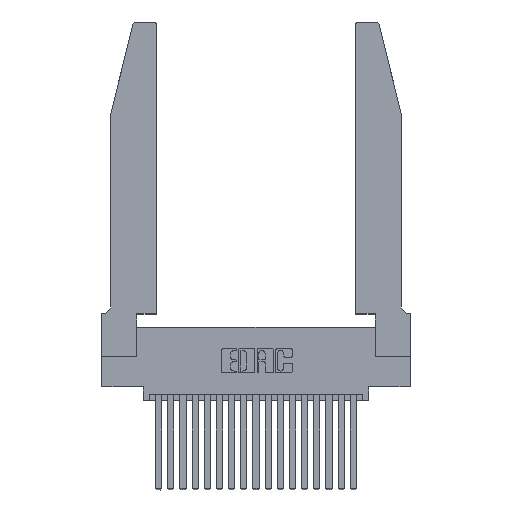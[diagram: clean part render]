
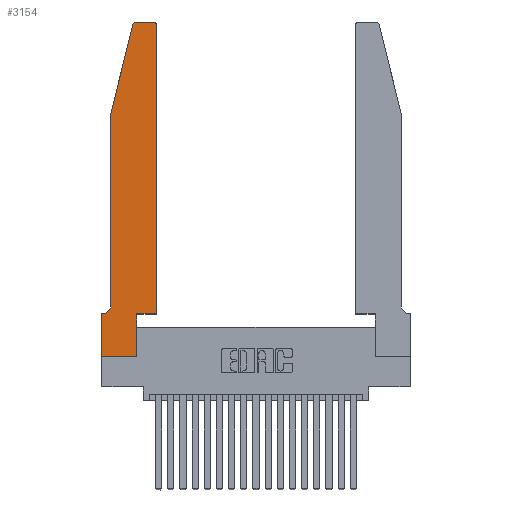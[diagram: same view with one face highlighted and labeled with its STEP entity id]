
A CAD part, top view. The second image highlights one B-rep face of the part: STEP entity #3154.
In plain terms, the highlighted planar face has unit normal (0, 0, 1).
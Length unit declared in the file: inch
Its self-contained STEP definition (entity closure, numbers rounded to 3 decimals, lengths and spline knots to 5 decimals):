
#36 = VECTOR ( 'NONE', #15393, 39.37008 ) ;
#44 = DIRECTION ( 'NONE',  ( 1., 0., 0. ) ) ;
#97 = CARTESIAN_POINT ( 'NONE',  ( 0.0055, 0.35, 0.37 ) ) ;
#299 = CIRCLE ( 'NONE', #5243, 0.07 ) ;
#672 = CARTESIAN_POINT ( 'NONE',  ( 0., 0., 0.37 ) ) ;
#752 = EDGE_CURVE ( 'NONE', #21136, #11259, #12921, .T. ) ;
#969 = CARTESIAN_POINT ( 'NONE',  ( 0.4505, 0.35, 0.37 ) ) ;
#1030 = VERTEX_POINT ( 'NONE', #6808 ) ;
#1181 = DIRECTION ( 'NONE',  ( 1., 0., 0. ) ) ;
#1696 = DIRECTION ( 'NONE',  ( 1., 0., 0. ) ) ;
#1903 = DIRECTION ( 'NONE',  ( -1., 0., 0. ) ) ;
#1952 = VECTOR ( 'NONE', #4539, 39.37008 ) ;
#2122 = VECTOR ( 'NONE', #17268, 39.37008 ) ;
#2132 = AXIS2_PLACEMENT_3D ( 'NONE', #18991, #7705, #6198 ) ;
#2528 = VECTOR ( 'NONE', #1696, 39.37008 ) ;
#2540 = CARTESIAN_POINT ( 'NONE',  ( 0.2865, 0., 0.37 ) ) ;
#2707 = LINE ( 'NONE', #16855, #19790 ) ;
#3154 = ADVANCED_FACE ( 'NONE', ( #4166 ), #10965, .T. ) ;
#3483 = DIRECTION ( 'NONE',  ( -1., 0., 0. ) ) ;
#3607 = VERTEX_POINT ( 'NONE', #16973 ) ;
#3768 = DIRECTION ( 'NONE',  ( 0., -1., 0. ) ) ;
#4088 = LINE ( 'NONE', #9942, #2528 ) ;
#4166 = FACE_OUTER_BOUND ( 'NONE', #20637, .T. ) ;
#4196 = VECTOR ( 'NONE', #15660, 39.37008 ) ;
#4365 = ORIENTED_EDGE ( 'NONE', *, *, #20532, .T. ) ;
#4539 = DIRECTION ( 'NONE',  ( -0.239, -0.971, 0. ) ) ;
#4566 = DIRECTION ( 'NONE',  ( 0., 0., 1. ) ) ;
#4737 = CARTESIAN_POINT ( 'NONE',  ( 0.4505, 0.35, 0.37 ) ) ;
#4977 = LINE ( 'NONE', #672, #4196 ) ;
#5243 = AXIS2_PLACEMENT_3D ( 'NONE', #11735, #13390, #3483 ) ;
#5324 = VECTOR ( 'NONE', #1903, 39.37008 ) ;
#5449 = ORIENTED_EDGE ( 'NONE', *, *, #10488, .T. ) ;
#5749 = VERTEX_POINT ( 'NONE', #17830 ) ;
#5934 = CARTESIAN_POINT ( 'NONE',  ( 0.25487, 2.72718, 0.37 ) ) ;
#6198 = DIRECTION ( 'NONE',  ( 1., 0., 0. ) ) ;
#6441 = ORIENTED_EDGE ( 'NONE', *, *, #20755, .T. ) ;
#6808 = CARTESIAN_POINT ( 'NONE',  ( 0.0755, 2., 0.37 ) ) ;
#7166 = CARTESIAN_POINT ( 'NONE',  ( 0.0755, 2., 0.37 ) ) ;
#7630 = CARTESIAN_POINT ( 'NONE',  ( 0.0755, 0.35, 0.37 ) ) ;
#7705 = DIRECTION ( 'NONE',  ( 0., 0., 1. ) ) ;
#7918 = VERTEX_POINT ( 'NONE', #9169 ) ;
#7986 = ORIENTED_EDGE ( 'NONE', *, *, #752, .T. ) ;
#8143 = LINE ( 'NONE', #12915, #1952 ) ;
#8164 = LINE ( 'NONE', #7630, #5324 ) ;
#8849 = EDGE_CURVE ( 'NONE', #10085, #20418, #20414, .T. ) ;
#9169 = CARTESIAN_POINT ( 'NONE',  ( 0., 0., 0.37 ) ) ;
#9395 = VERTEX_POINT ( 'NONE', #18356 ) ;
#9600 = DIRECTION ( 'NONE',  ( -1., 0., 0. ) ) ;
#9942 = CARTESIAN_POINT ( 'NONE',  ( 0., 0., 0.37 ) ) ;
#10085 = VERTEX_POINT ( 'NONE', #15931 ) ;
#10093 = EDGE_CURVE ( 'NONE', #17256, #16939, #8164, .T. ) ;
#10488 = EDGE_CURVE ( 'NONE', #20418, #1030, #8143, .T. ) ;
#10801 = ORIENTED_EDGE ( 'NONE', *, *, #17318, .T. ) ;
#10965 = PLANE ( 'NONE',  #2132 ) ;
#11007 = CARTESIAN_POINT ( 'NONE',  ( 0., 0.35, 0.37 ) ) ;
#11152 = EDGE_CURVE ( 'NONE', #3607, #10085, #2707, .T. ) ;
#11259 = VERTEX_POINT ( 'NONE', #14756 ) ;
#11735 = CARTESIAN_POINT ( 'NONE',  ( 0.0055, 0.42, 0.37 ) ) ;
#12325 = VECTOR ( 'NONE', #3768, 39.37008 ) ;
#12838 = LINE ( 'NONE', #7166, #12325 ) ;
#12915 = CARTESIAN_POINT ( 'NONE',  ( 0.0755, 2., 0.37 ) ) ;
#12921 = LINE ( 'NONE', #15279, #14443 ) ;
#13390 = DIRECTION ( 'NONE',  ( 0., 0., -1. ) ) ;
#13433 = AXIS2_PLACEMENT_3D ( 'NONE', #14601, #19554, #44 ) ;
#14248 = AXIS2_PLACEMENT_3D ( 'NONE', #19527, #4566, #1181 ) ;
#14443 = VECTOR ( 'NONE', #16862, 39.37008 ) ;
#14601 = CARTESIAN_POINT ( 'NONE',  ( 0.4205, 2.72, 0.37 ) ) ;
#14756 = CARTESIAN_POINT ( 'NONE',  ( 0.2865, 0.35, 0.37 ) ) ;
#14759 = ORIENTED_EDGE ( 'NONE', *, *, #16573, .T. ) ;
#15279 = CARTESIAN_POINT ( 'NONE',  ( 0.2865, 0.35, 0.37 ) ) ;
#15393 = DIRECTION ( 'NONE',  ( 1., 0., 0. ) ) ;
#15625 = ORIENTED_EDGE ( 'NONE', *, *, #8849, .T. ) ;
#15660 = DIRECTION ( 'NONE',  ( 0., -1., 0. ) ) ;
#15722 = ORIENTED_EDGE ( 'NONE', *, *, #20921, .T. ) ;
#15931 = CARTESIAN_POINT ( 'NONE',  ( 0.284, 2.75, 0.37 ) ) ;
#16549 = LINE ( 'NONE', #18294, #36 ) ;
#16573 = EDGE_CURVE ( 'NONE', #7918, #21136, #4088, .T. ) ;
#16817 = CIRCLE ( 'NONE', #13433, 0.03 ) ;
#16855 = CARTESIAN_POINT ( 'NONE',  ( 0.2605, 2.75, 0.37 ) ) ;
#16862 = DIRECTION ( 'NONE',  ( 0., 1., 0. ) ) ;
#16939 = VERTEX_POINT ( 'NONE', #11007 ) ;
#16973 = CARTESIAN_POINT ( 'NONE',  ( 0.4205, 2.75, 0.37 ) ) ;
#17256 = VERTEX_POINT ( 'NONE', #97 ) ;
#17268 = DIRECTION ( 'NONE',  ( 0., 1., 0. ) ) ;
#17318 = EDGE_CURVE ( 'NONE', #1030, #5749, #12838, .T. ) ;
#17830 = CARTESIAN_POINT ( 'NONE',  ( 0.0755, 0.42, 0.37 ) ) ;
#18162 = ORIENTED_EDGE ( 'NONE', *, *, #10093, .T. ) ;
#18294 = CARTESIAN_POINT ( 'NONE',  ( 0.4505, 0.35, 0.37 ) ) ;
#18356 = CARTESIAN_POINT ( 'NONE',  ( 0.4505, 2.72, 0.37 ) ) ;
#18650 = ORIENTED_EDGE ( 'NONE', *, *, #11152, .T. ) ;
#18991 = CARTESIAN_POINT ( 'NONE',  ( 0., 0.35, 0.37 ) ) ;
#19034 = VERTEX_POINT ( 'NONE', #4737 ) ;
#19220 = ORIENTED_EDGE ( 'NONE', *, *, #19930, .T. ) ;
#19527 = CARTESIAN_POINT ( 'NONE',  ( 0.284, 2.72, 0.37 ) ) ;
#19554 = DIRECTION ( 'NONE',  ( 0., 0., 1. ) ) ;
#19790 = VECTOR ( 'NONE', #9600, 39.37008 ) ;
#19930 = EDGE_CURVE ( 'NONE', #16939, #7918, #4977, .T. ) ;
#20414 = CIRCLE ( 'NONE', #14248, 0.03 ) ;
#20418 = VERTEX_POINT ( 'NONE', #5934 ) ;
#20492 = LINE ( 'NONE', #969, #2122 ) ;
#20532 = EDGE_CURVE ( 'NONE', #19034, #9395, #20492, .T. ) ;
#20566 = ORIENTED_EDGE ( 'NONE', *, *, #20879, .T. ) ;
#20637 = EDGE_LOOP ( 'NONE', ( #18650, #15625, #5449, #10801, #20566, #18162, #19220, #14759, #7986, #15722, #4365, #6441 ) ) ;
#20755 = EDGE_CURVE ( 'NONE', #9395, #3607, #16817, .T. ) ;
#20879 = EDGE_CURVE ( 'NONE', #5749, #17256, #299, .T. ) ;
#20921 = EDGE_CURVE ( 'NONE', #11259, #19034, #16549, .T. ) ;
#21136 = VERTEX_POINT ( 'NONE', #2540 ) ;
